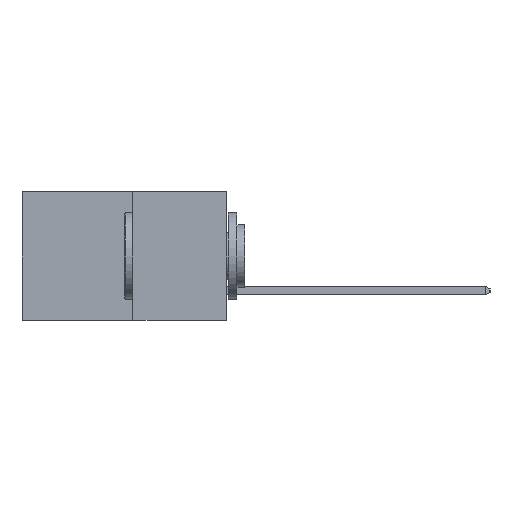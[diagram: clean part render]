
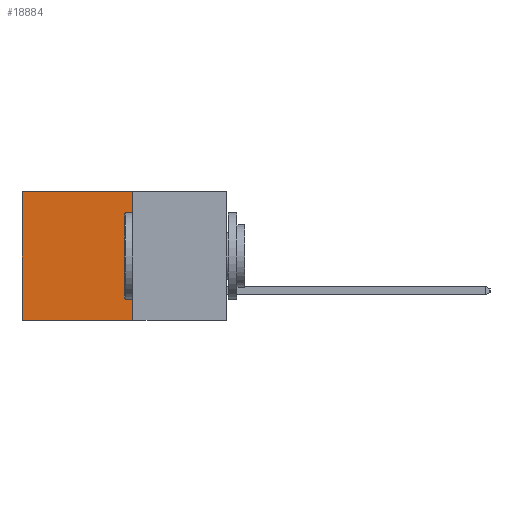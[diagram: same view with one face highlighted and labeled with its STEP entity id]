
A CAD part, left-side view. The second image highlights one B-rep face of the part: STEP entity #18884.
In plain terms, the highlighted planar face has unit normal (-1, 0, 0).
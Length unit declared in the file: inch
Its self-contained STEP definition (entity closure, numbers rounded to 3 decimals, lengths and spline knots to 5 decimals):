
#1331 = VECTOR ( 'NONE', #3954, 39.37008 ) ;
#1390 = CARTESIAN_POINT ( 'NONE',  ( 0.277, 0.27, -0.37 ) ) ;
#1866 = CARTESIAN_POINT ( 'NONE',  ( 0.277, 0.59, 0. ) ) ;
#2090 = DIRECTION ( 'NONE',  ( 0., 0., -1. ) ) ;
#2391 = FACE_OUTER_BOUND ( 'NONE', #24151, .T. ) ;
#3397 = VECTOR ( 'NONE', #2090, 39.37008 ) ;
#3468 = DIRECTION ( 'NONE',  ( 0., 0., -1. ) ) ;
#3852 = DIRECTION ( 'NONE',  ( 0., 0., -1. ) ) ;
#3954 = DIRECTION ( 'NONE',  ( 0., 1., 0. ) ) ;
#5268 = ORIENTED_EDGE ( 'NONE', *, *, #8731, .F. ) ;
#5288 = VECTOR ( 'NONE', #22114, 39.37008 ) ;
#5394 = VERTEX_POINT ( 'NONE', #11150 ) ;
#5494 = LINE ( 'NONE', #25482, #25163 ) ;
#8363 = CARTESIAN_POINT ( 'NONE',  ( 0.277, 0.27, -0.37 ) ) ;
#8731 = EDGE_CURVE ( 'NONE', #5394, #18869, #20459, .T. ) ;
#9024 = ORIENTED_EDGE ( 'NONE', *, *, #25308, .T. ) ;
#11150 = CARTESIAN_POINT ( 'NONE',  ( 0.277, 0.27, -0.37 ) ) ;
#11301 = EDGE_CURVE ( 'NONE', #16222, #5394, #5494, .T. ) ;
#11495 = CARTESIAN_POINT ( 'NONE',  ( 0.277, 0.59, -0.37 ) ) ;
#13064 = EDGE_CURVE ( 'NONE', #19189, #18869, #19326, .T. ) ;
#15293 = CARTESIAN_POINT ( 'NONE',  ( 0.277, 0.27, 0. ) ) ;
#15434 = DIRECTION ( 'NONE',  ( 1., 0., 0. ) ) ;
#15866 = CARTESIAN_POINT ( 'NONE',  ( 0.277, 0.27, 0. ) ) ;
#16074 = ORIENTED_EDGE ( 'NONE', *, *, #11301, .F. ) ;
#16222 = VERTEX_POINT ( 'NONE', #15293 ) ;
#16728 = LINE ( 'NONE', #15866, #1331 ) ;
#18869 = VERTEX_POINT ( 'NONE', #11495 ) ;
#18884 = ADVANCED_FACE ( 'NONE', ( #2391 ), #23241, .F. ) ;
#19116 = AXIS2_PLACEMENT_3D ( 'NONE', #1390, #15434, #3468 ) ;
#19189 = VERTEX_POINT ( 'NONE', #1866 ) ;
#19326 = LINE ( 'NONE', #23886, #3397 ) ;
#20286 = ORIENTED_EDGE ( 'NONE', *, *, #13064, .T. ) ;
#20459 = LINE ( 'NONE', #8363, #5288 ) ;
#22114 = DIRECTION ( 'NONE',  ( 0., 1., 0. ) ) ;
#23241 = PLANE ( 'NONE',  #19116 ) ;
#23886 = CARTESIAN_POINT ( 'NONE',  ( 0.277, 0.59, -0.37 ) ) ;
#24151 = EDGE_LOOP ( 'NONE', ( #20286, #5268, #16074, #9024 ) ) ;
#25163 = VECTOR ( 'NONE', #3852, 39.37008 ) ;
#25308 = EDGE_CURVE ( 'NONE', #16222, #19189, #16728, .T. ) ;
#25482 = CARTESIAN_POINT ( 'NONE',  ( 0.277, 0.27, -0.37 ) ) ;
